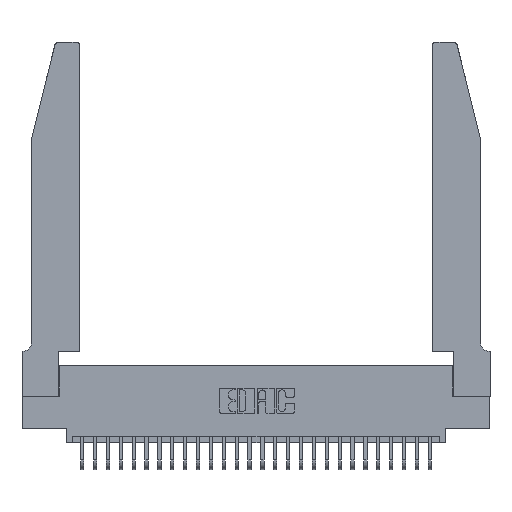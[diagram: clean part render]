
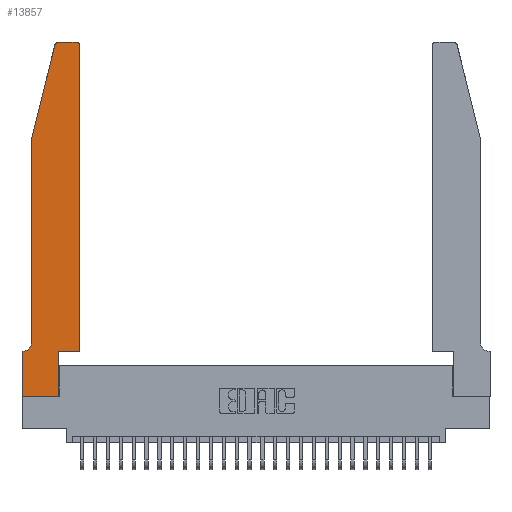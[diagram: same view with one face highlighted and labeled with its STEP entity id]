
A CAD part, top view. The second image highlights one B-rep face of the part: STEP entity #13857.
In plain terms, the highlighted planar face has unit normal (0, 0, 1).
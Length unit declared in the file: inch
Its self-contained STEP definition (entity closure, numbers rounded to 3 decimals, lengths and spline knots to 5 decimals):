
#435 = DIRECTION ( 'NONE',  ( -1., 0., 0. ) ) ;
#633 = VERTEX_POINT ( 'NONE', #14200 ) ;
#1374 = ORIENTED_EDGE ( 'NONE', *, *, #6082, .T. ) ;
#1608 = DIRECTION ( 'NONE',  ( 1., 0., 0. ) ) ;
#1839 = EDGE_CURVE ( 'NONE', #26590, #5023, #4105, .T. ) ;
#1893 = LINE ( 'NONE', #25546, #19951 ) ;
#2181 = VERTEX_POINT ( 'NONE', #7607 ) ;
#2435 = VERTEX_POINT ( 'NONE', #22515 ) ;
#2638 = EDGE_CURVE ( 'NONE', #2181, #633, #1893, .T. ) ;
#2709 = CARTESIAN_POINT ( 'NONE',  ( 0.0755, 0.35, 0.37 ) ) ;
#2884 = DIRECTION ( 'NONE',  ( -0.239, -0.971, 0. ) ) ;
#3144 = CARTESIAN_POINT ( 'NONE',  ( 0.2865, 0., 0.37 ) ) ;
#3338 = CARTESIAN_POINT ( 'NONE',  ( 0., 0., 0.37 ) ) ;
#4105 = CIRCLE ( 'NONE', #7154, 0.07 ) ;
#4448 = DIRECTION ( 'NONE',  ( 0., -1., 0. ) ) ;
#5023 = VERTEX_POINT ( 'NONE', #16687 ) ;
#5484 = DIRECTION ( 'NONE',  ( 0., 0., 1. ) ) ;
#5591 = VECTOR ( 'NONE', #4448, 39.37008 ) ;
#6082 = EDGE_CURVE ( 'NONE', #19205, #23486, #21929, .T. ) ;
#6870 = VECTOR ( 'NONE', #27719, 39.37008 ) ;
#7149 = CIRCLE ( 'NONE', #9565, 0.03 ) ;
#7154 = AXIS2_PLACEMENT_3D ( 'NONE', #20511, #26988, #23323 ) ;
#7195 = EDGE_CURVE ( 'NONE', #27621, #27321, #10363, .T. ) ;
#7506 = VECTOR ( 'NONE', #16716, 39.37008 ) ;
#7607 = CARTESIAN_POINT ( 'NONE',  ( 0.4505, 0.35, 0.37 ) ) ;
#7642 = ORIENTED_EDGE ( 'NONE', *, *, #12385, .T. ) ;
#7905 = CARTESIAN_POINT ( 'NONE',  ( 0.0755, 2., 0.37 ) ) ;
#8346 = ORIENTED_EDGE ( 'NONE', *, *, #7195, .T. ) ;
#8464 = ORIENTED_EDGE ( 'NONE', *, *, #21613, .T. ) ;
#8793 = ORIENTED_EDGE ( 'NONE', *, *, #29376, .T. ) ;
#8913 = CARTESIAN_POINT ( 'NONE',  ( 0.2605, 2.75, 0.37 ) ) ;
#9389 = AXIS2_PLACEMENT_3D ( 'NONE', #19561, #5484, #21933 ) ;
#9509 = VECTOR ( 'NONE', #435, 39.37008 ) ;
#9565 = AXIS2_PLACEMENT_3D ( 'NONE', #27721, #13644, #30051 ) ;
#9774 = LINE ( 'NONE', #10590, #15307 ) ;
#10363 = LINE ( 'NONE', #18534, #5591 ) ;
#10476 = EDGE_CURVE ( 'NONE', #2435, #24826, #25613, .T. ) ;
#10577 = ORIENTED_EDGE ( 'NONE', *, *, #2638, .T. ) ;
#10590 = CARTESIAN_POINT ( 'NONE',  ( 0., 0., 0.37 ) ) ;
#10899 = EDGE_CURVE ( 'NONE', #18324, #26590, #25582, .T. ) ;
#11885 = CARTESIAN_POINT ( 'NONE',  ( 0.25487, 2.72718, 0.37 ) ) ;
#11952 = CIRCLE ( 'NONE', #9389, 0.03 ) ;
#12154 = EDGE_CURVE ( 'NONE', #24826, #18786, #7149, .T. ) ;
#12385 = EDGE_CURVE ( 'NONE', #23486, #2181, #19277, .T. ) ;
#12584 = LINE ( 'NONE', #28649, #23609 ) ;
#13304 = CARTESIAN_POINT ( 'NONE',  ( 0., 0.35, 0.37 ) ) ;
#13644 = DIRECTION ( 'NONE',  ( 0., 0., 1. ) ) ;
#13857 = ADVANCED_FACE ( 'NONE', ( #16886 ), #22695, .T. ) ;
#14200 = CARTESIAN_POINT ( 'NONE',  ( 0.4505, 2.72, 0.37 ) ) ;
#14508 = CARTESIAN_POINT ( 'NONE',  ( 0.2865, 0.35, 0.37 ) ) ;
#14514 = AXIS2_PLACEMENT_3D ( 'NONE', #13304, #15660, #1608 ) ;
#14551 = CARTESIAN_POINT ( 'NONE',  ( 0.284, 2.75, 0.37 ) ) ;
#15307 = VECTOR ( 'NONE', #29326, 39.37008 ) ;
#15660 = DIRECTION ( 'NONE',  ( 0., 0., 1. ) ) ;
#15752 = LINE ( 'NONE', #2709, #9509 ) ;
#16687 = CARTESIAN_POINT ( 'NONE',  ( 0.0055, 0.35, 0.37 ) ) ;
#16716 = DIRECTION ( 'NONE',  ( 1., 0., 0. ) ) ;
#16886 = FACE_OUTER_BOUND ( 'NONE', #28684, .T. ) ;
#17573 = ORIENTED_EDGE ( 'NONE', *, *, #12154, .T. ) ;
#18256 = CARTESIAN_POINT ( 'NONE',  ( 0.0755, 2., 0.37 ) ) ;
#18324 = VERTEX_POINT ( 'NONE', #7905 ) ;
#18387 = DIRECTION ( 'NONE',  ( 0., 1., 0. ) ) ;
#18534 = CARTESIAN_POINT ( 'NONE',  ( 0., 0., 0.37 ) ) ;
#18612 = VECTOR ( 'NONE', #25345, 39.37008 ) ;
#18786 = VERTEX_POINT ( 'NONE', #11885 ) ;
#19124 = ORIENTED_EDGE ( 'NONE', *, *, #10476, .T. ) ;
#19205 = VERTEX_POINT ( 'NONE', #3144 ) ;
#19277 = LINE ( 'NONE', #28409, #7506 ) ;
#19561 = CARTESIAN_POINT ( 'NONE',  ( 0.4205, 2.72, 0.37 ) ) ;
#19951 = VECTOR ( 'NONE', #27880, 39.37008 ) ;
#20511 = CARTESIAN_POINT ( 'NONE',  ( 0.0055, 0.42, 0.37 ) ) ;
#21613 = EDGE_CURVE ( 'NONE', #5023, #27621, #15752, .T. ) ;
#21929 = LINE ( 'NONE', #30040, #27395 ) ;
#21933 = DIRECTION ( 'NONE',  ( 1., 0., 0. ) ) ;
#22515 = CARTESIAN_POINT ( 'NONE',  ( 0.4205, 2.75, 0.37 ) ) ;
#22695 = PLANE ( 'NONE',  #14514 ) ;
#22821 = ORIENTED_EDGE ( 'NONE', *, *, #10899, .T. ) ;
#23323 = DIRECTION ( 'NONE',  ( -1., 0., 0. ) ) ;
#23486 = VERTEX_POINT ( 'NONE', #14508 ) ;
#23609 = VECTOR ( 'NONE', #2884, 39.37008 ) ;
#24135 = EDGE_CURVE ( 'NONE', #633, #2435, #11952, .T. ) ;
#24826 = VERTEX_POINT ( 'NONE', #14551 ) ;
#25345 = DIRECTION ( 'NONE',  ( 0., -1., 0. ) ) ;
#25546 = CARTESIAN_POINT ( 'NONE',  ( 0.4505, 0.35, 0.37 ) ) ;
#25582 = LINE ( 'NONE', #18256, #18612 ) ;
#25613 = LINE ( 'NONE', #8913, #6870 ) ;
#25833 = EDGE_CURVE ( 'NONE', #18786, #18324, #12584, .T. ) ;
#26286 = CARTESIAN_POINT ( 'NONE',  ( 0.0755, 0.42, 0.37 ) ) ;
#26504 = ORIENTED_EDGE ( 'NONE', *, *, #1839, .T. ) ;
#26590 = VERTEX_POINT ( 'NONE', #26286 ) ;
#26988 = DIRECTION ( 'NONE',  ( 0., 0., -1. ) ) ;
#27321 = VERTEX_POINT ( 'NONE', #3338 ) ;
#27395 = VECTOR ( 'NONE', #18387, 39.37008 ) ;
#27621 = VERTEX_POINT ( 'NONE', #30389 ) ;
#27719 = DIRECTION ( 'NONE',  ( -1., 0., 0. ) ) ;
#27721 = CARTESIAN_POINT ( 'NONE',  ( 0.284, 2.72, 0.37 ) ) ;
#27880 = DIRECTION ( 'NONE',  ( 0., 1., 0. ) ) ;
#28318 = ORIENTED_EDGE ( 'NONE', *, *, #25833, .T. ) ;
#28409 = CARTESIAN_POINT ( 'NONE',  ( 0.4505, 0.35, 0.37 ) ) ;
#28649 = CARTESIAN_POINT ( 'NONE',  ( 0.0755, 2., 0.37 ) ) ;
#28684 = EDGE_LOOP ( 'NONE', ( #19124, #17573, #28318, #22821, #26504, #8464, #8346, #8793, #1374, #7642, #10577, #29268 ) ) ;
#29268 = ORIENTED_EDGE ( 'NONE', *, *, #24135, .T. ) ;
#29326 = DIRECTION ( 'NONE',  ( 1., 0., 0. ) ) ;
#29376 = EDGE_CURVE ( 'NONE', #27321, #19205, #9774, .T. ) ;
#30040 = CARTESIAN_POINT ( 'NONE',  ( 0.2865, 0.35, 0.37 ) ) ;
#30051 = DIRECTION ( 'NONE',  ( 1., 0., 0. ) ) ;
#30389 = CARTESIAN_POINT ( 'NONE',  ( 0., 0.35, 0.37 ) ) ;
